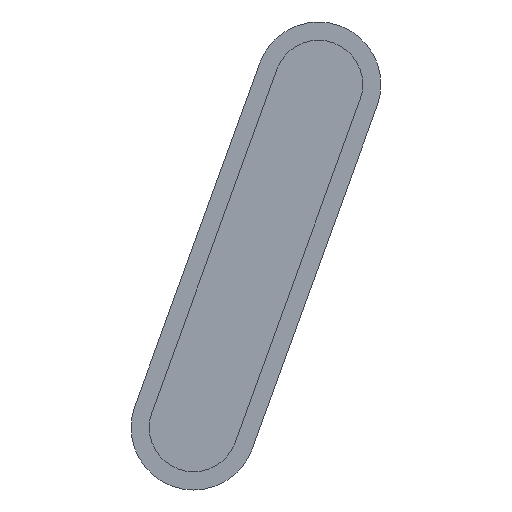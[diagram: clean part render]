
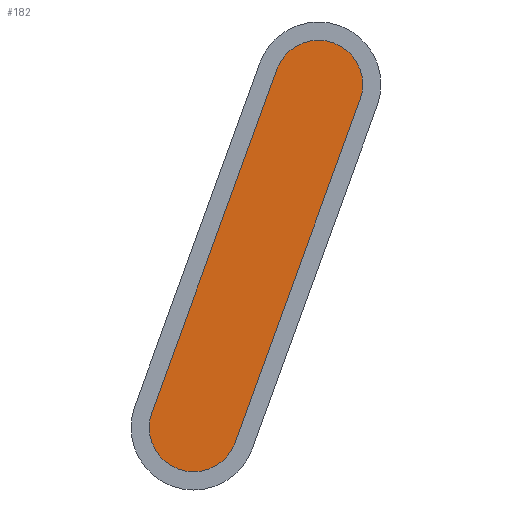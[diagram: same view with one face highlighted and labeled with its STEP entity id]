
A CAD part, front view. The second image highlights one B-rep face of the part: STEP entity #182.
In plain terms, the highlighted planar face has unit normal (0, -1, 0).
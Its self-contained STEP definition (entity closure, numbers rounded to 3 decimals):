
#18=PLANE('',#211);
#27=FACE_OUTER_BOUND('',#38,.T.);
#38=EDGE_LOOP('',(#142,#143,#144,#145));
#50=LINE('',#293,#66);
#52=LINE('',#298,#68);
#66=VECTOR('',#236,10.);
#68=VECTOR('',#240,10.);
#79=CIRCLE('',#205,4.85);
#81=CIRCLE('',#210,4.85);
#88=VERTEX_POINT('',#283);
#89=VERTEX_POINT('',#285);
#91=VERTEX_POINT('',#291);
#93=VERTEX_POINT('',#297);
#104=EDGE_CURVE('',#89,#88,#79,.T.);
#108=EDGE_CURVE('',#88,#91,#50,.T.);
#110=EDGE_CURVE('',#93,#89,#52,.T.);
#113=EDGE_CURVE('',#91,#93,#81,.T.);
#142=ORIENTED_EDGE('',*,*,#108,.T.);
#143=ORIENTED_EDGE('',*,*,#113,.T.);
#144=ORIENTED_EDGE('',*,*,#110,.T.);
#145=ORIENTED_EDGE('',*,*,#104,.T.);
#182=ADVANCED_FACE('',(#27),#18,.F.);
#205=AXIS2_PLACEMENT_3D('',#286,#229,#230);
#210=AXIS2_PLACEMENT_3D('',#302,#246,#247);
#211=AXIS2_PLACEMENT_3D('',#303,#248,#249);
#229=DIRECTION('center_axis',(0.,-1.,0.));
#230=DIRECTION('ref_axis',(-0.94,0.,0.342));
#236=DIRECTION('',(-0.342,0.,-0.94));
#240=DIRECTION('',(0.342,0.,0.94));
#246=DIRECTION('center_axis',(0.,-1.,0.));
#247=DIRECTION('ref_axis',(0.94,0.,-0.342));
#248=DIRECTION('center_axis',(0.,1.,0.));
#249=DIRECTION('ref_axis',(-1.,0.,0.));
#283=CARTESIAN_POINT('',(39.52,-12.192,26.645));
#285=CARTESIAN_POINT('',(48.635,-12.192,23.328));
#286=CARTESIAN_POINT('Origin',(44.077,-12.192,24.987));
#291=CARTESIAN_POINT('',(25.839,-12.192,-10.942));
#293=CARTESIAN_POINT('',(36.099,-12.192,17.248));
#297=CARTESIAN_POINT('',(34.954,-12.192,-14.26));
#298=CARTESIAN_POINT('',(38.374,-12.192,-4.863));
#302=CARTESIAN_POINT('Origin',(30.396,-12.192,-12.601));
#303=CARTESIAN_POINT('Origin',(37.237,-12.192,6.193));
